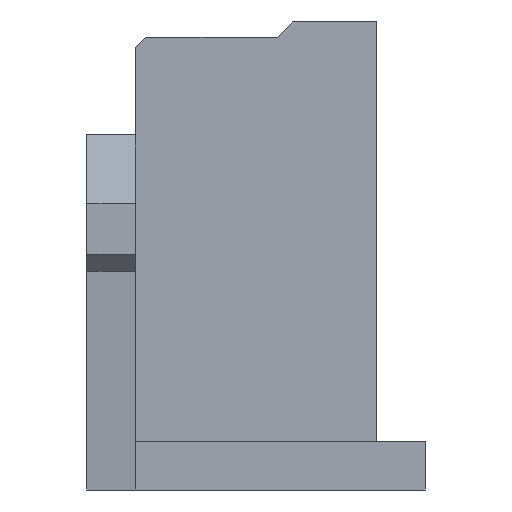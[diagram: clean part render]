
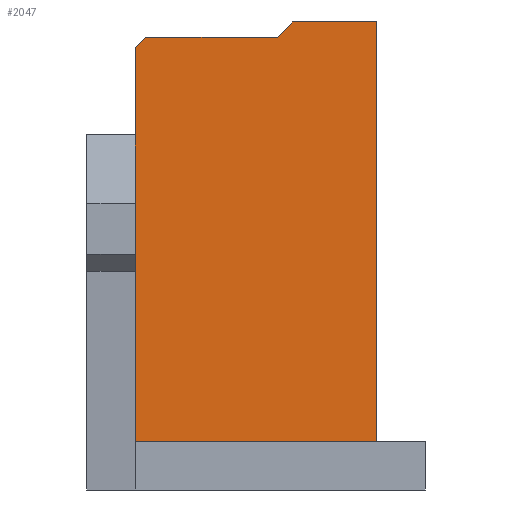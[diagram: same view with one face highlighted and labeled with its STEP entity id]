
A CAD part, left-side view. The second image highlights one B-rep face of the part: STEP entity #2047.
In plain terms, the highlighted planar face has unit normal (-1, 0, 0).
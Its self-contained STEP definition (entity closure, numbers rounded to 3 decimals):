
#173 = DIRECTION ( 'NONE',  ( 0., -0.707, 0.707 ) ) ;
#216 = LINE ( 'NONE', #3389, #7283 ) ;
#255 = DIRECTION ( 'NONE',  ( 0., 0., -1. ) ) ;
#424 = CARTESIAN_POINT ( 'NONE',  ( -12.85, 4., 3.448 ) ) ;
#518 = EDGE_CURVE ( 'NONE', #4551, #3981, #1718, .T. ) ;
#596 = EDGE_CURVE ( 'NONE', #7900, #1318, #4365, .T. ) ;
#611 = VERTEX_POINT ( 'NONE', #7336 ) ;
#809 = ORIENTED_EDGE ( 'NONE', *, *, #518, .F. ) ;
#1318 = VERTEX_POINT ( 'NONE', #1541 ) ;
#1428 = LINE ( 'NONE', #3837, #7847 ) ;
#1541 = CARTESIAN_POINT ( 'NONE',  ( -12.85, 0., 3.875 ) ) ;
#1710 = CARTESIAN_POINT ( 'NONE',  ( -12.85, 0., -3.075 ) ) ;
#1718 = LINE ( 'NONE', #2862, #7959 ) ;
#1755 = CARTESIAN_POINT ( 'NONE',  ( -12.85, 3.823, 3.625 ) ) ;
#1911 = DIRECTION ( 'NONE',  ( 0., -1., 0. ) ) ;
#1947 = EDGE_CURVE ( 'NONE', #1318, #5697, #216, .T. ) ;
#2047 = ADVANCED_FACE ( 'NONE', ( #4387 ), #7969, .F. ) ;
#2128 = VERTEX_POINT ( 'NONE', #4346 ) ;
#2321 = CARTESIAN_POINT ( 'NONE',  ( -12.85, 4., -3.875 ) ) ;
#2359 = LINE ( 'NONE', #2321, #4253 ) ;
#2858 = EDGE_LOOP ( 'NONE', ( #4905, #4989, #3821, #4502, #5497, #809, #3845 ) ) ;
#2862 = CARTESIAN_POINT ( 'NONE',  ( -12.85, 3.823, 3.625 ) ) ;
#2946 = VECTOR ( 'NONE', #1911, 1000. ) ;
#3002 = DIRECTION ( 'NONE',  ( 1., 0., 0. ) ) ;
#3052 = LINE ( 'NONE', #4839, #2946 ) ;
#3389 = CARTESIAN_POINT ( 'NONE',  ( -12.85, 0., 3.875 ) ) ;
#3821 = ORIENTED_EDGE ( 'NONE', *, *, #596, .F. ) ;
#3837 = CARTESIAN_POINT ( 'NONE',  ( -12.85, 1.4, 3.875 ) ) ;
#3845 = ORIENTED_EDGE ( 'NONE', *, *, #5678, .F. ) ;
#3981 = VERTEX_POINT ( 'NONE', #1755 ) ;
#4077 = EDGE_CURVE ( 'NONE', #2128, #7900, #1428, .T. ) ;
#4202 = DIRECTION ( 'NONE',  ( 0., -0.707, 0.707 ) ) ;
#4253 = VECTOR ( 'NONE', #5377, 1000. ) ;
#4285 = DIRECTION ( 'NONE',  ( 0., -1., 0. ) ) ;
#4346 = CARTESIAN_POINT ( 'NONE',  ( -12.85, 1.65, 3.625 ) ) ;
#4365 = LINE ( 'NONE', #4853, #5110 ) ;
#4387 = FACE_OUTER_BOUND ( 'NONE', #2858, .T. ) ;
#4502 = ORIENTED_EDGE ( 'NONE', *, *, #4077, .F. ) ;
#4551 = VERTEX_POINT ( 'NONE', #424 ) ;
#4839 = CARTESIAN_POINT ( 'NONE',  ( -12.85, 0., -3.075 ) ) ;
#4853 = CARTESIAN_POINT ( 'NONE',  ( -12.85, 1.4, 3.875 ) ) ;
#4905 = ORIENTED_EDGE ( 'NONE', *, *, #5571, .T. ) ;
#4943 = AXIS2_PLACEMENT_3D ( 'NONE', #6703, #3002, #6129 ) ;
#4989 = ORIENTED_EDGE ( 'NONE', *, *, #1947, .F. ) ;
#5110 = VECTOR ( 'NONE', #4285, 1000. ) ;
#5174 = DIRECTION ( 'NONE',  ( 0., -1., 0. ) ) ;
#5377 = DIRECTION ( 'NONE',  ( 0., 0., 1. ) ) ;
#5440 = VECTOR ( 'NONE', #5174, 1000. ) ;
#5497 = ORIENTED_EDGE ( 'NONE', *, *, #7095, .F. ) ;
#5571 = EDGE_CURVE ( 'NONE', #611, #5697, #3052, .T. ) ;
#5678 = EDGE_CURVE ( 'NONE', #611, #4551, #2359, .T. ) ;
#5697 = VERTEX_POINT ( 'NONE', #1710 ) ;
#5700 = CARTESIAN_POINT ( 'NONE',  ( -12.85, 1.4, 3.875 ) ) ;
#6129 = DIRECTION ( 'NONE',  ( 0., 0., -1. ) ) ;
#6474 = CARTESIAN_POINT ( 'NONE',  ( -12.85, 3.823, 3.625 ) ) ;
#6511 = LINE ( 'NONE', #6474, #5440 ) ;
#6703 = CARTESIAN_POINT ( 'NONE',  ( -12.85, 0., 0. ) ) ;
#7095 = EDGE_CURVE ( 'NONE', #3981, #2128, #6511, .T. ) ;
#7283 = VECTOR ( 'NONE', #255, 1000. ) ;
#7336 = CARTESIAN_POINT ( 'NONE',  ( -12.85, 4., -3.075 ) ) ;
#7847 = VECTOR ( 'NONE', #173, 1000. ) ;
#7900 = VERTEX_POINT ( 'NONE', #5700 ) ;
#7959 = VECTOR ( 'NONE', #4202, 1000. ) ;
#7969 = PLANE ( 'NONE',  #4943 ) ;
